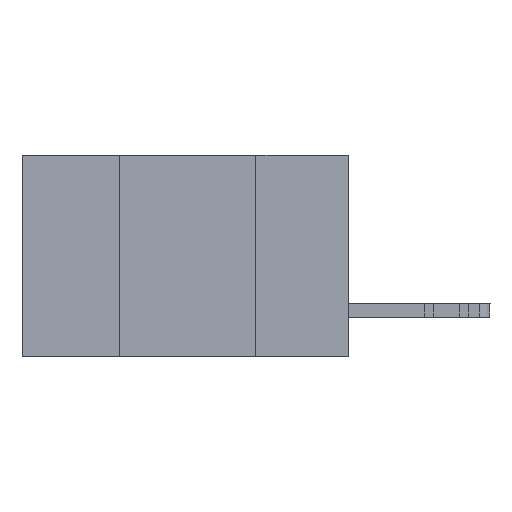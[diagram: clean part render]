
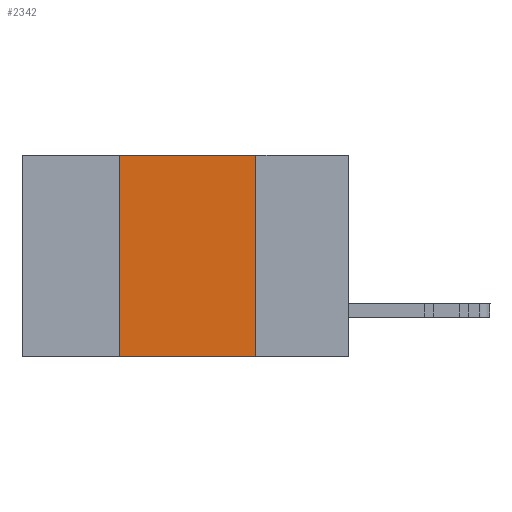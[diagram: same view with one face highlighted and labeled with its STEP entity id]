
A CAD part, left-side view. The second image highlights one B-rep face of the part: STEP entity #2342.
In plain terms, the highlighted planar face has unit normal (-1, 0, 0).
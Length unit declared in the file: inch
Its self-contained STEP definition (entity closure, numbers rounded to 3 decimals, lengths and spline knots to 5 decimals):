
#79 = LINE ( 'NONE', #13432, #5773 ) ;
#465 = EDGE_LOOP ( 'NONE', ( #10947, #28538, #577, #16822 ) ) ;
#577 = ORIENTED_EDGE ( 'NONE', *, *, #28911, .F. ) ;
#946 = DIRECTION ( 'NONE',  ( 0., 0., 1. ) ) ;
#2342 = ADVANCED_FACE ( 'NONE', ( #19141 ), #30979, .F. ) ;
#4049 = VERTEX_POINT ( 'NONE', #16698 ) ;
#4551 = AXIS2_PLACEMENT_3D ( 'NONE', #11727, #14115, #16555 ) ;
#4869 = LINE ( 'NONE', #10270, #23401 ) ;
#4971 = EDGE_CURVE ( 'NONE', #4049, #29730, #79, .T. ) ;
#5773 = VECTOR ( 'NONE', #13543, 39.37008 ) ;
#6528 = CARTESIAN_POINT ( 'NONE',  ( 0., 0.42, 0. ) ) ;
#8994 = CARTESIAN_POINT ( 'NONE',  ( 0., 0.17, -0.37 ) ) ;
#10270 = CARTESIAN_POINT ( 'NONE',  ( 0., 0.42, 0. ) ) ;
#10947 = ORIENTED_EDGE ( 'NONE', *, *, #4971, .F. ) ;
#11727 = CARTESIAN_POINT ( 'NONE',  ( 0., 0.6, 0. ) ) ;
#13432 = CARTESIAN_POINT ( 'NONE',  ( 0., 0.17, 0. ) ) ;
#13543 = DIRECTION ( 'NONE',  ( 0., 0., -1. ) ) ;
#14115 = DIRECTION ( 'NONE',  ( 1., 0., 0. ) ) ;
#15002 = VERTEX_POINT ( 'NONE', #6528 ) ;
#15144 = VECTOR ( 'NONE', #16213, 39.37008 ) ;
#16213 = DIRECTION ( 'NONE',  ( 0., -1., 0. ) ) ;
#16555 = DIRECTION ( 'NONE',  ( 0., 0., -1. ) ) ;
#16698 = CARTESIAN_POINT ( 'NONE',  ( 0., 0.17, 0. ) ) ;
#16822 = ORIENTED_EDGE ( 'NONE', *, *, #18287, .T. ) ;
#18287 = EDGE_CURVE ( 'NONE', #30363, #29730, #29466, .T. ) ;
#18644 = CARTESIAN_POINT ( 'NONE',  ( 0., 0.6, -0.37 ) ) ;
#19141 = FACE_OUTER_BOUND ( 'NONE', #465, .T. ) ;
#20352 = CARTESIAN_POINT ( 'NONE',  ( 0., 0.42, -0.37 ) ) ;
#23122 = LINE ( 'NONE', #23248, #23515 ) ;
#23248 = CARTESIAN_POINT ( 'NONE',  ( 0., 0.6, 0. ) ) ;
#23401 = VECTOR ( 'NONE', #946, 39.37008 ) ;
#23515 = VECTOR ( 'NONE', #28102, 39.37008 ) ;
#27339 = EDGE_CURVE ( 'NONE', #15002, #4049, #23122, .T. ) ;
#28102 = DIRECTION ( 'NONE',  ( 0., -1., 0. ) ) ;
#28538 = ORIENTED_EDGE ( 'NONE', *, *, #27339, .F. ) ;
#28911 = EDGE_CURVE ( 'NONE', #30363, #15002, #4869, .T. ) ;
#29466 = LINE ( 'NONE', #18644, #15144 ) ;
#29730 = VERTEX_POINT ( 'NONE', #8994 ) ;
#30363 = VERTEX_POINT ( 'NONE', #20352 ) ;
#30979 = PLANE ( 'NONE',  #4551 ) ;
